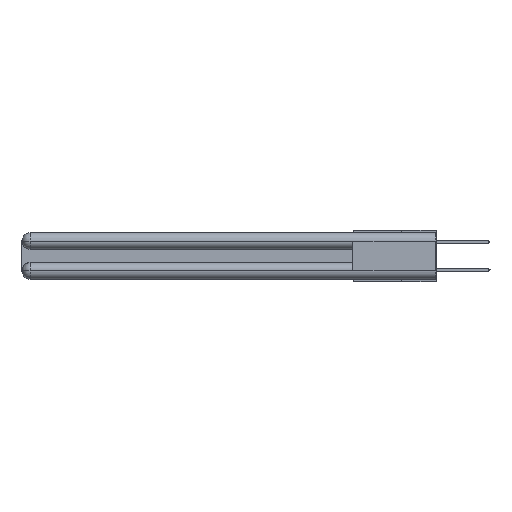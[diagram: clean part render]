
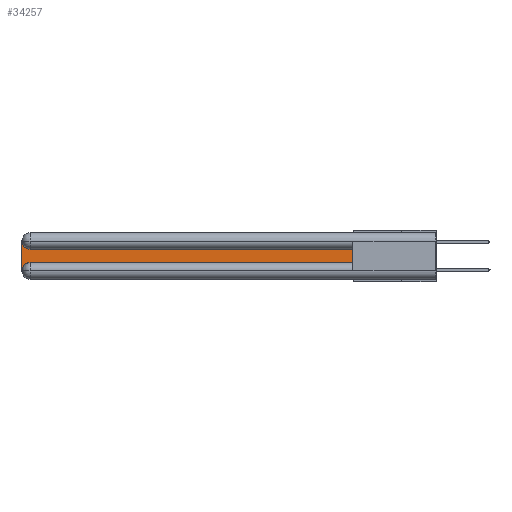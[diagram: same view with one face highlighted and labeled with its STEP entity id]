
A CAD part, left-side view. The second image highlights one B-rep face of the part: STEP entity #34257.
In plain terms, the highlighted planar face has unit normal (-1, 0, 0).
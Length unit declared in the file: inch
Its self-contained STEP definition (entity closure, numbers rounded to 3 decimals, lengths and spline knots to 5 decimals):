
#105 = ORIENTED_EDGE ( 'NONE', *, *, #35534, .T. ) ;
#1111 = DIRECTION ( 'NONE',  ( 0., 0., -1. ) ) ;
#3098 = AXIS2_PLACEMENT_3D ( 'NONE', #23680, #7784, #1111 ) ;
#3262 = FACE_OUTER_BOUND ( 'NONE', #28162, .T. ) ;
#4629 = VECTOR ( 'NONE', #33934, 39.37008 ) ;
#4933 = CIRCLE ( 'NONE', #27634, 0.06 ) ;
#5280 = DIRECTION ( 'NONE',  ( 0., 1., 0. ) ) ;
#7784 = DIRECTION ( 'NONE',  ( 1., 0., 0. ) ) ;
#7897 = VERTEX_POINT ( 'NONE', #17469 ) ;
#9060 = VECTOR ( 'NONE', #12788, 39.37008 ) ;
#10471 = ORIENTED_EDGE ( 'NONE', *, *, #34470, .T. ) ;
#10702 = LINE ( 'NONE', #31169, #4629 ) ;
#12788 = DIRECTION ( 'NONE',  ( 0., 0., 1. ) ) ;
#12931 = VERTEX_POINT ( 'NONE', #23289 ) ;
#13225 = CARTESIAN_POINT ( 'NONE',  ( 0.075, 2.94, -0.1225 ) ) ;
#13260 = CARTESIAN_POINT ( 'NONE',  ( 0.075, 3., -0.2175 ) ) ;
#13717 = VECTOR ( 'NONE', #5280, 39.37008 ) ;
#14085 = CARTESIAN_POINT ( 'NONE',  ( 0.075, 2.94, -0.2175 ) ) ;
#14407 = CARTESIAN_POINT ( 'NONE',  ( 0.075, 2.94, -0.0625 ) ) ;
#15269 = VERTEX_POINT ( 'NONE', #13225 ) ;
#16050 = DIRECTION ( 'NONE',  ( 0., 0., -1. ) ) ;
#16438 = LINE ( 'NONE', #32032, #9060 ) ;
#16569 = ORIENTED_EDGE ( 'NONE', *, *, #20121, .T. ) ;
#16928 = CIRCLE ( 'NONE', #3098, 0.06 ) ;
#17036 = VERTEX_POINT ( 'NONE', #32160 ) ;
#17105 = CARTESIAN_POINT ( 'NONE',  ( 0.075, 3., -0.1225 ) ) ;
#17469 = CARTESIAN_POINT ( 'NONE',  ( 0.075, 3., -0.0625 ) ) ;
#19222 = EDGE_CURVE ( 'NONE', #17036, #34056, #16928, .T. ) ;
#20091 = DIRECTION ( 'NONE',  ( 0., 0., -1. ) ) ;
#20121 = EDGE_CURVE ( 'NONE', #12931, #23058, #16438, .T. ) ;
#21146 = AXIS2_PLACEMENT_3D ( 'NONE', #17105, #22666, #22917 ) ;
#21884 = CARTESIAN_POINT ( 'NONE',  ( 0.075, 0.6, -0.1225 ) ) ;
#22666 = DIRECTION ( 'NONE',  ( 1., 0., 0. ) ) ;
#22917 = DIRECTION ( 'NONE',  ( 0., 0., -1. ) ) ;
#23058 = VERTEX_POINT ( 'NONE', #30307 ) ;
#23289 = CARTESIAN_POINT ( 'NONE',  ( 0.075, 0.6, -0.2175 ) ) ;
#23680 = CARTESIAN_POINT ( 'NONE',  ( 0.075, 2.94, -0.2775 ) ) ;
#25506 = VECTOR ( 'NONE', #16050, 39.37008 ) ;
#25575 = PLANE ( 'NONE',  #21146 ) ;
#27634 = AXIS2_PLACEMENT_3D ( 'NONE', #14407, #33627, #20091 ) ;
#27650 = EDGE_CURVE ( 'NONE', #7897, #17036, #27669, .T. ) ;
#27669 = LINE ( 'NONE', #13260, #25506 ) ;
#28162 = EDGE_LOOP ( 'NONE', ( #10471, #105, #35415, #33032, #29813, #16569 ) ) ;
#29813 = ORIENTED_EDGE ( 'NONE', *, *, #32628, .T. ) ;
#30307 = CARTESIAN_POINT ( 'NONE',  ( 0.075, 0.6, -0.1225 ) ) ;
#31169 = CARTESIAN_POINT ( 'NONE',  ( 0.075, 0.6, -0.2175 ) ) ;
#32032 = CARTESIAN_POINT ( 'NONE',  ( 0.075, 0.6, -0.2175 ) ) ;
#32160 = CARTESIAN_POINT ( 'NONE',  ( 0.075, 3., -0.2775 ) ) ;
#32628 = EDGE_CURVE ( 'NONE', #34056, #12931, #10702, .T. ) ;
#33032 = ORIENTED_EDGE ( 'NONE', *, *, #19222, .T. ) ;
#33627 = DIRECTION ( 'NONE',  ( 1., 0., 0. ) ) ;
#33934 = DIRECTION ( 'NONE',  ( 0., -1., 0. ) ) ;
#34039 = LINE ( 'NONE', #21884, #13717 ) ;
#34056 = VERTEX_POINT ( 'NONE', #14085 ) ;
#34257 = ADVANCED_FACE ( 'NONE', ( #3262 ), #25575, .F. ) ;
#34470 = EDGE_CURVE ( 'NONE', #23058, #15269, #34039, .T. ) ;
#35415 = ORIENTED_EDGE ( 'NONE', *, *, #27650, .T. ) ;
#35534 = EDGE_CURVE ( 'NONE', #15269, #7897, #4933, .T. ) ;
